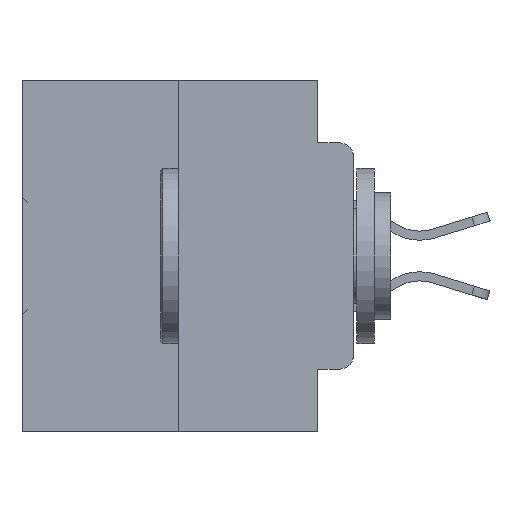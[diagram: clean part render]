
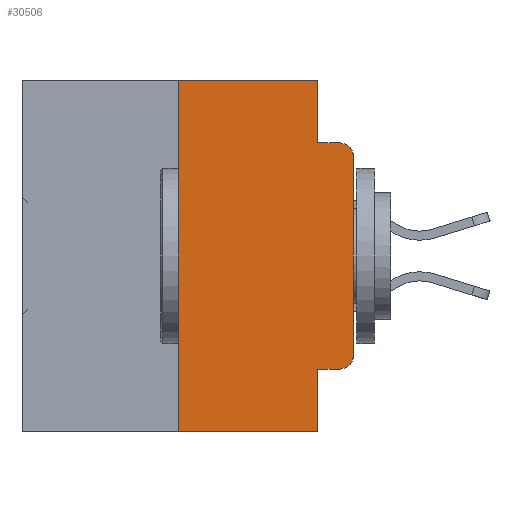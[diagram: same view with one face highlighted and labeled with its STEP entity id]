
A CAD part, left-side view. The second image highlights one B-rep face of the part: STEP entity #30506.
In plain terms, the highlighted planar face has unit normal (-1, 0, 0).
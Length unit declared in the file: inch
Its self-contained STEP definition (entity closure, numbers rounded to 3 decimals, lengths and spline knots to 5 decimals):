
#695 = EDGE_LOOP ( 'NONE', ( #11791, #5312, #26238, #35404, #10835, #881, #30632, #10103, #11828, #26681 ) ) ;
#881 = ORIENTED_EDGE ( 'NONE', *, *, #30680, .F. ) ;
#1153 = CARTESIAN_POINT ( 'NONE',  ( 0., 0.051, -0.4115 ) ) ;
#1429 = LINE ( 'NONE', #1153, #30279 ) ;
#1901 = EDGE_CURVE ( 'NONE', #35518, #18147, #25779, .T. ) ;
#2085 = FACE_OUTER_BOUND ( 'NONE', #695, .T. ) ;
#2517 = CARTESIAN_POINT ( 'NONE',  ( 0., 0., 0. ) ) ;
#2556 = CARTESIAN_POINT ( 'NONE',  ( 0., 0.02, -0.0885 ) ) ;
#2703 = DIRECTION ( 'NONE',  ( 0., 0., -1. ) ) ;
#2873 = LINE ( 'NONE', #2517, #24252 ) ;
#3192 = DIRECTION ( 'NONE',  ( -1., 0., 0. ) ) ;
#3807 = EDGE_CURVE ( 'NONE', #18147, #12460, #8698, .T. ) ;
#4306 = VECTOR ( 'NONE', #35855, 39.37008 ) ;
#4376 = CARTESIAN_POINT ( 'NONE',  ( 0., 0.473, -0.5 ) ) ;
#4412 = VECTOR ( 'NONE', #7302, 39.37008 ) ;
#4443 = VECTOR ( 'NONE', #2703, 39.37008 ) ;
#4499 = DIRECTION ( 'NONE',  ( 0., -1., 0. ) ) ;
#5034 = AXIS2_PLACEMENT_3D ( 'NONE', #9907, #35147, #18460 ) ;
#5185 = LINE ( 'NONE', #13500, #4306 ) ;
#5312 = ORIENTED_EDGE ( 'NONE', *, *, #11265, .T. ) ;
#5643 = VERTEX_POINT ( 'NONE', #11021 ) ;
#5734 = DIRECTION ( 'NONE',  ( -1., 0., 0. ) ) ;
#7302 = DIRECTION ( 'NONE',  ( 0., 0., -1. ) ) ;
#7349 = CARTESIAN_POINT ( 'NONE',  ( 0., 0.051, 0. ) ) ;
#8188 = VERTEX_POINT ( 'NONE', #16819 ) ;
#8632 = VERTEX_POINT ( 'NONE', #29954 ) ;
#8698 = LINE ( 'NONE', #34204, #30048 ) ;
#9615 = DIRECTION ( 'NONE',  ( 0., -1., 0. ) ) ;
#9907 = CARTESIAN_POINT ( 'NONE',  ( 0., 0.473, 0. ) ) ;
#10103 = ORIENTED_EDGE ( 'NONE', *, *, #28818, .F. ) ;
#10347 = EDGE_CURVE ( 'NONE', #34421, #8632, #22279, .T. ) ;
#10835 = ORIENTED_EDGE ( 'NONE', *, *, #31885, .F. ) ;
#11021 = CARTESIAN_POINT ( 'NONE',  ( 0., 0., -0.1085 ) ) ;
#11247 = CARTESIAN_POINT ( 'NONE',  ( 0., 0.051, 0. ) ) ;
#11265 = EDGE_CURVE ( 'NONE', #5643, #12460, #15629, .T. ) ;
#11791 = ORIENTED_EDGE ( 'NONE', *, *, #13116, .T. ) ;
#11808 = CARTESIAN_POINT ( 'NONE',  ( 0., 0.051, -0.0885 ) ) ;
#11828 = ORIENTED_EDGE ( 'NONE', *, *, #19481, .T. ) ;
#11936 = EDGE_CURVE ( 'NONE', #8188, #20992, #15121, .T. ) ;
#12460 = VERTEX_POINT ( 'NONE', #2556 ) ;
#12483 = AXIS2_PLACEMENT_3D ( 'NONE', #19951, #3192, #22724 ) ;
#13116 = EDGE_CURVE ( 'NONE', #20992, #5643, #2873, .T. ) ;
#13500 = CARTESIAN_POINT ( 'NONE',  ( 0., 0.25, 0. ) ) ;
#14794 = VECTOR ( 'NONE', #29290, 39.37008 ) ;
#15121 = CIRCLE ( 'NONE', #12483, 0.02 ) ;
#15561 = VERTEX_POINT ( 'NONE', #16003 ) ;
#15629 = CIRCLE ( 'NONE', #25837, 0.02 ) ;
#16003 = CARTESIAN_POINT ( 'NONE',  ( 0., 0.25, 0. ) ) ;
#16819 = CARTESIAN_POINT ( 'NONE',  ( 0., 0.02, -0.4115 ) ) ;
#17433 = CARTESIAN_POINT ( 'NONE',  ( 0., 0.25, -0.5 ) ) ;
#18147 = VERTEX_POINT ( 'NONE', #11808 ) ;
#18460 = DIRECTION ( 'NONE',  ( 0., 0., -1. ) ) ;
#19242 = DIRECTION ( 'NONE',  ( 0., 0., 1. ) ) ;
#19481 = EDGE_CURVE ( 'NONE', #30766, #8188, #1429, .T. ) ;
#19669 = CARTESIAN_POINT ( 'NONE',  ( 0., 0., -0.3915 ) ) ;
#19951 = CARTESIAN_POINT ( 'NONE',  ( 0., 0.02, -0.3915 ) ) ;
#20992 = VERTEX_POINT ( 'NONE', #19669 ) ;
#21207 = CARTESIAN_POINT ( 'NONE',  ( 0., 0.473, 0. ) ) ;
#22279 = LINE ( 'NONE', #4376, #14794 ) ;
#22303 = LINE ( 'NONE', #21207, #29687 ) ;
#22348 = CARTESIAN_POINT ( 'NONE',  ( 0., 0.051, -0.4115 ) ) ;
#22428 = CARTESIAN_POINT ( 'NONE',  ( 0., 0.02, -0.1085 ) ) ;
#22724 = DIRECTION ( 'NONE',  ( 0., 0., -1. ) ) ;
#23930 = PLANE ( 'NONE',  #5034 ) ;
#24252 = VECTOR ( 'NONE', #19242, 39.37008 ) ;
#25213 = DIRECTION ( 'NONE',  ( 0., 0., -1. ) ) ;
#25779 = LINE ( 'NONE', #7349, #4412 ) ;
#25837 = AXIS2_PLACEMENT_3D ( 'NONE', #22428, #5734, #25213 ) ;
#26238 = ORIENTED_EDGE ( 'NONE', *, *, #3807, .F. ) ;
#26681 = ORIENTED_EDGE ( 'NONE', *, *, #11936, .T. ) ;
#28818 = EDGE_CURVE ( 'NONE', #30766, #8632, #34970, .T. ) ;
#29290 = DIRECTION ( 'NONE',  ( 0., -1., 0. ) ) ;
#29687 = VECTOR ( 'NONE', #4499, 39.37008 ) ;
#29954 = CARTESIAN_POINT ( 'NONE',  ( 0., 0.051, -0.5 ) ) ;
#30048 = VECTOR ( 'NONE', #33329, 39.37008 ) ;
#30279 = VECTOR ( 'NONE', #9615, 39.37008 ) ;
#30506 = ADVANCED_FACE ( 'NONE', ( #2085 ), #23930, .F. ) ;
#30632 = ORIENTED_EDGE ( 'NONE', *, *, #10347, .T. ) ;
#30633 = CARTESIAN_POINT ( 'NONE',  ( 0., 0.051, 0. ) ) ;
#30680 = EDGE_CURVE ( 'NONE', #34421, #15561, #5185, .T. ) ;
#30766 = VERTEX_POINT ( 'NONE', #22348 ) ;
#31885 = EDGE_CURVE ( 'NONE', #15561, #35518, #22303, .T. ) ;
#33329 = DIRECTION ( 'NONE',  ( 0., -1., 0. ) ) ;
#34204 = CARTESIAN_POINT ( 'NONE',  ( 0., 0.051, -0.0885 ) ) ;
#34421 = VERTEX_POINT ( 'NONE', #17433 ) ;
#34970 = LINE ( 'NONE', #30633, #4443 ) ;
#35147 = DIRECTION ( 'NONE',  ( 1., 0., 0. ) ) ;
#35404 = ORIENTED_EDGE ( 'NONE', *, *, #1901, .F. ) ;
#35518 = VERTEX_POINT ( 'NONE', #11247 ) ;
#35855 = DIRECTION ( 'NONE',  ( 0., 0., 1. ) ) ;
